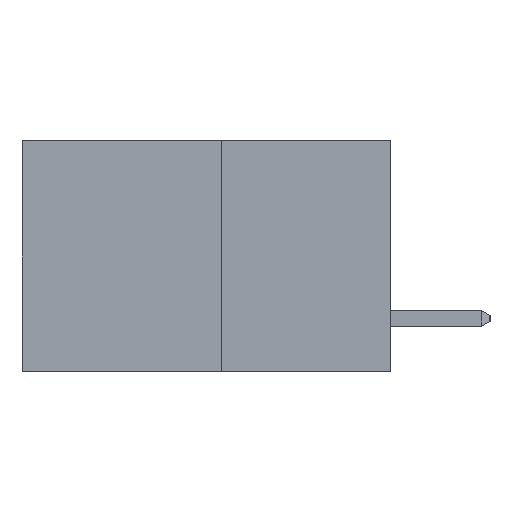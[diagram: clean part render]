
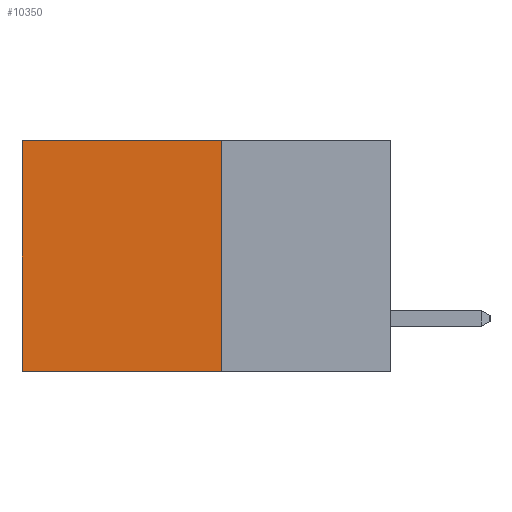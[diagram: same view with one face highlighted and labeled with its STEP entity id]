
A CAD part, left-side view. The second image highlights one B-rep face of the part: STEP entity #10350.
In plain terms, the highlighted planar face has unit normal (-1, 0, 0).
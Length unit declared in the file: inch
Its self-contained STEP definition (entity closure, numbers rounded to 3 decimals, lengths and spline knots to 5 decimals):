
#953 = CARTESIAN_POINT ( 'NONE',  ( 0.277, 0.27, -0.37 ) ) ;
#987 = VERTEX_POINT ( 'NONE', #13040 ) ;
#1001 = DIRECTION ( 'NONE',  ( 0., 0., -1. ) ) ;
#1028 = CARTESIAN_POINT ( 'NONE',  ( 0.277, 0.27, -0.37 ) ) ;
#1976 = ORIENTED_EDGE ( 'NONE', *, *, #9876, .T. ) ;
#2646 = ORIENTED_EDGE ( 'NONE', *, *, #6064, .F. ) ;
#3256 = DIRECTION ( 'NONE',  ( 0., 0., -1. ) ) ;
#3457 = DIRECTION ( 'NONE',  ( 0., 1., 0. ) ) ;
#3568 = ORIENTED_EDGE ( 'NONE', *, *, #9558, .T. ) ;
#3662 = LINE ( 'NONE', #6176, #6430 ) ;
#3789 = CARTESIAN_POINT ( 'NONE',  ( 0.277, 0.27, -0.37 ) ) ;
#3948 = CARTESIAN_POINT ( 'NONE',  ( 0.277, 0.27, -0.37 ) ) ;
#4305 = FACE_OUTER_BOUND ( 'NONE', #11114, .T. ) ;
#4631 = CARTESIAN_POINT ( 'NONE',  ( 0.277, 0.59, -0.37 ) ) ;
#4874 = VECTOR ( 'NONE', #3457, 39.37008 ) ;
#4973 = LINE ( 'NONE', #4631, #12897 ) ;
#5165 = EDGE_CURVE ( 'NONE', #11454, #6060, #13130, .T. ) ;
#5688 = DIRECTION ( 'NONE',  ( 0., 0., -1. ) ) ;
#6060 = VERTEX_POINT ( 'NONE', #3948 ) ;
#6064 = EDGE_CURVE ( 'NONE', #6060, #987, #10229, .T. ) ;
#6072 = CARTESIAN_POINT ( 'NONE',  ( 0.277, 0.27, 0. ) ) ;
#6132 = DIRECTION ( 'NONE',  ( 0., 1., 0. ) ) ;
#6176 = CARTESIAN_POINT ( 'NONE',  ( 0.277, 0.27, 0. ) ) ;
#6430 = VECTOR ( 'NONE', #6132, 39.37008 ) ;
#8438 = PLANE ( 'NONE',  #11565 ) ;
#8454 = ORIENTED_EDGE ( 'NONE', *, *, #5165, .F. ) ;
#9411 = DIRECTION ( 'NONE',  ( 1., 0., 0. ) ) ;
#9558 = EDGE_CURVE ( 'NONE', #11454, #11714, #3662, .T. ) ;
#9876 = EDGE_CURVE ( 'NONE', #11714, #987, #4973, .T. ) ;
#10229 = LINE ( 'NONE', #3789, #4874 ) ;
#10252 = VECTOR ( 'NONE', #1001, 39.37008 ) ;
#10350 = ADVANCED_FACE ( 'NONE', ( #4305 ), #8438, .F. ) ;
#11114 = EDGE_LOOP ( 'NONE', ( #1976, #2646, #8454, #3568 ) ) ;
#11454 = VERTEX_POINT ( 'NONE', #6072 ) ;
#11565 = AXIS2_PLACEMENT_3D ( 'NONE', #1028, #9411, #3256 ) ;
#11714 = VERTEX_POINT ( 'NONE', #12403 ) ;
#12403 = CARTESIAN_POINT ( 'NONE',  ( 0.277, 0.59, 0. ) ) ;
#12897 = VECTOR ( 'NONE', #5688, 39.37008 ) ;
#13040 = CARTESIAN_POINT ( 'NONE',  ( 0.277, 0.59, -0.37 ) ) ;
#13130 = LINE ( 'NONE', #953, #10252 ) ;
